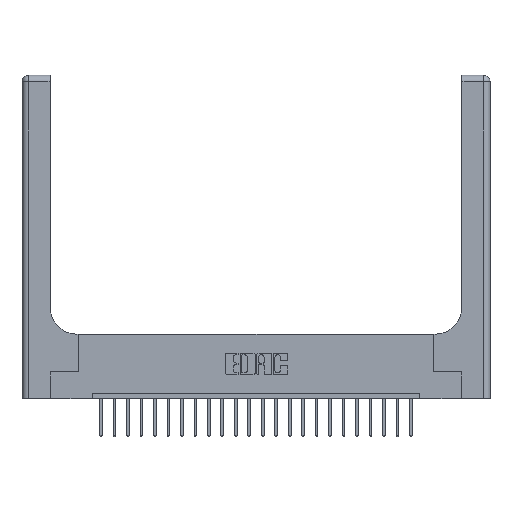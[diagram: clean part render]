
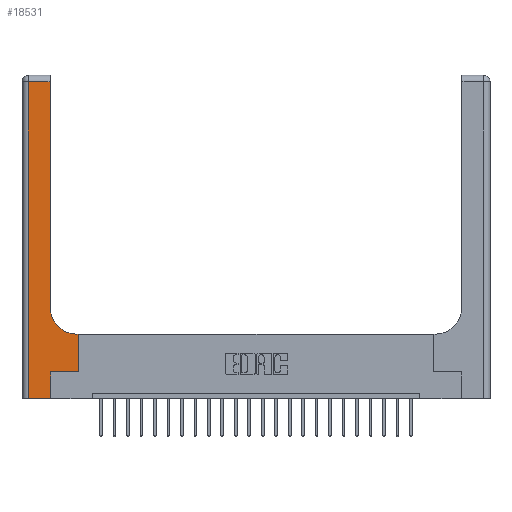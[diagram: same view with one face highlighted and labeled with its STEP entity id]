
A CAD part, top view. The second image highlights one B-rep face of the part: STEP entity #18531.
In plain terms, the highlighted planar face has unit normal (0, 0, 1).
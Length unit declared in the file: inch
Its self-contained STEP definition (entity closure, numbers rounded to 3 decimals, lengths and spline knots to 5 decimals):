
#145 = LINE ( 'NONE', #10680, #3689 ) ;
#203 = EDGE_CURVE ( 'NONE', #6638, #12280, #17254, .T. ) ;
#394 = VECTOR ( 'NONE', #19355, 39.37008 ) ;
#1015 = DIRECTION ( 'NONE',  ( 0., 1., 0. ) ) ;
#1155 = EDGE_CURVE ( 'NONE', #21124, #18646, #145, .T. ) ;
#1479 = CARTESIAN_POINT ( 'NONE',  ( 0.06, 3., 0.37 ) ) ;
#1770 = LINE ( 'NONE', #14174, #18365 ) ;
#1894 = EDGE_CURVE ( 'NONE', #16365, #17034, #18754, .T. ) ;
#1958 = ORIENTED_EDGE ( 'NONE', *, *, #21531, .T. ) ;
#1966 = EDGE_CURVE ( 'NONE', #18646, #6638, #15968, .T. ) ;
#2172 = CIRCLE ( 'NONE', #9583, 0.25 ) ;
#2242 = AXIS2_PLACEMENT_3D ( 'NONE', #18260, #14910, #11540 ) ;
#2979 = CARTESIAN_POINT ( 'NONE',  ( 0.51, 0.6, 0.37 ) ) ;
#3191 = CARTESIAN_POINT ( 'NONE',  ( 0.528, 0.6, 0.37 ) ) ;
#3296 = ORIENTED_EDGE ( 'NONE', *, *, #14252, .T. ) ;
#3689 = VECTOR ( 'NONE', #5206, 39.37008 ) ;
#5206 = DIRECTION ( 'NONE',  ( -1., 0., 0. ) ) ;
#5337 = DIRECTION ( 'NONE',  ( -1., 0., 0. ) ) ;
#5502 = EDGE_CURVE ( 'NONE', #20108, #21124, #8191, .T. ) ;
#6288 = FACE_OUTER_BOUND ( 'NONE', #12359, .T. ) ;
#6638 = VERTEX_POINT ( 'NONE', #10793 ) ;
#6903 = CARTESIAN_POINT ( 'NONE',  ( 0.26, 2.94, 0.37 ) ) ;
#7195 = CARTESIAN_POINT ( 'NONE',  ( 0.26, 0.85, 0.37 ) ) ;
#7551 = CARTESIAN_POINT ( 'NONE',  ( 0.265, 0., 0.37 ) ) ;
#7722 = DIRECTION ( 'NONE',  ( 1., 0., 0. ) ) ;
#8097 = DIRECTION ( 'NONE',  ( 1., 0., 0. ) ) ;
#8191 = LINE ( 'NONE', #8423, #12360 ) ;
#8423 = CARTESIAN_POINT ( 'NONE',  ( 0.26, 3., 0.37 ) ) ;
#8457 = CARTESIAN_POINT ( 'NONE',  ( 0.265, 0., 0.37 ) ) ;
#8868 = LINE ( 'NONE', #7551, #21293 ) ;
#9158 = CARTESIAN_POINT ( 'NONE',  ( 0.528, 0.25, 0.37 ) ) ;
#9280 = CARTESIAN_POINT ( 'NONE',  ( 0.265, 0.25, 0.37 ) ) ;
#9583 = AXIS2_PLACEMENT_3D ( 'NONE', #15372, #20627, #10159 ) ;
#9731 = VECTOR ( 'NONE', #8097, 39.37008 ) ;
#10159 = DIRECTION ( 'NONE',  ( 1., 0., 0. ) ) ;
#10507 = ORIENTED_EDGE ( 'NONE', *, *, #21223, .T. ) ;
#10680 = CARTESIAN_POINT ( 'NONE',  ( 0., 2.94, 0.37 ) ) ;
#10793 = CARTESIAN_POINT ( 'NONE',  ( 0.06, 0., 0.37 ) ) ;
#11003 = EDGE_CURVE ( 'NONE', #17034, #13604, #1770, .T. ) ;
#11195 = LINE ( 'NONE', #19953, #19797 ) ;
#11540 = DIRECTION ( 'NONE',  ( -1., 0., 0. ) ) ;
#11910 = CARTESIAN_POINT ( 'NONE',  ( 0.528, 0.25, 0.37 ) ) ;
#12280 = VERTEX_POINT ( 'NONE', #8457 ) ;
#12359 = EDGE_LOOP ( 'NONE', ( #16500, #12892, #19020, #19418, #1958, #10507, #15483, #14059, #3296 ) ) ;
#12360 = VECTOR ( 'NONE', #1015, 39.37008 ) ;
#12892 = ORIENTED_EDGE ( 'NONE', *, *, #1155, .T. ) ;
#13043 = PLANE ( 'NONE',  #2242 ) ;
#13604 = VERTEX_POINT ( 'NONE', #2979 ) ;
#14059 = ORIENTED_EDGE ( 'NONE', *, *, #11003, .T. ) ;
#14174 = CARTESIAN_POINT ( 'NONE',  ( 0.26, 0.6, 0.37 ) ) ;
#14252 = EDGE_CURVE ( 'NONE', #13604, #20108, #2172, .T. ) ;
#14910 = DIRECTION ( 'NONE',  ( 0., 0., -1. ) ) ;
#15029 = CARTESIAN_POINT ( 'NONE',  ( 0.06, 2.94, 0.37 ) ) ;
#15276 = DIRECTION ( 'NONE',  ( 0., 1., 0. ) ) ;
#15372 = CARTESIAN_POINT ( 'NONE',  ( 0.51, 0.85, 0.37 ) ) ;
#15483 = ORIENTED_EDGE ( 'NONE', *, *, #1894, .T. ) ;
#15968 = LINE ( 'NONE', #1479, #394 ) ;
#16365 = VERTEX_POINT ( 'NONE', #9158 ) ;
#16500 = ORIENTED_EDGE ( 'NONE', *, *, #5502, .T. ) ;
#16915 = CARTESIAN_POINT ( 'NONE',  ( 0., 0., 0.37 ) ) ;
#17034 = VERTEX_POINT ( 'NONE', #3191 ) ;
#17254 = LINE ( 'NONE', #16915, #9731 ) ;
#17630 = VERTEX_POINT ( 'NONE', #9280 ) ;
#18260 = CARTESIAN_POINT ( 'NONE',  ( 0., 3., 0.37 ) ) ;
#18365 = VECTOR ( 'NONE', #5337, 39.37008 ) ;
#18531 = ADVANCED_FACE ( 'NONE', ( #6288 ), #13043, .F. ) ;
#18646 = VERTEX_POINT ( 'NONE', #15029 ) ;
#18754 = LINE ( 'NONE', #11910, #21910 ) ;
#19020 = ORIENTED_EDGE ( 'NONE', *, *, #1966, .T. ) ;
#19355 = DIRECTION ( 'NONE',  ( 0., -1., 0. ) ) ;
#19418 = ORIENTED_EDGE ( 'NONE', *, *, #203, .T. ) ;
#19797 = VECTOR ( 'NONE', #7722, 39.37008 ) ;
#19893 = DIRECTION ( 'NONE',  ( 0., 1., 0. ) ) ;
#19953 = CARTESIAN_POINT ( 'NONE',  ( 0.265, 0.25, 0.37 ) ) ;
#20108 = VERTEX_POINT ( 'NONE', #7195 ) ;
#20627 = DIRECTION ( 'NONE',  ( 0., 0., -1. ) ) ;
#21124 = VERTEX_POINT ( 'NONE', #6903 ) ;
#21223 = EDGE_CURVE ( 'NONE', #17630, #16365, #11195, .T. ) ;
#21293 = VECTOR ( 'NONE', #19893, 39.37008 ) ;
#21531 = EDGE_CURVE ( 'NONE', #12280, #17630, #8868, .T. ) ;
#21910 = VECTOR ( 'NONE', #15276, 39.37008 ) ;
